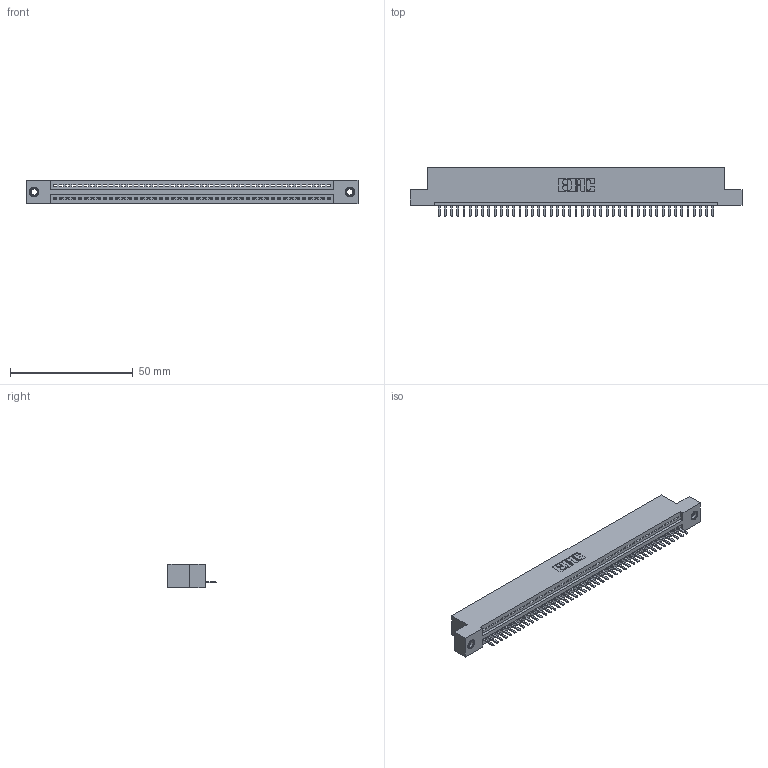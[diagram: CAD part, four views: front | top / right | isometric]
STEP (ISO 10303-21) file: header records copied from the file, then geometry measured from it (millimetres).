
FILE_DESCRIPTION (( 'STEP AP203' ), '1' );
FILE_NAME ('395-045-520-107.STEP', '2019-10-22T17:28:25', ( '' ), ( '' ), 'SwSTEP 2.0', 'SolidWorks 2016', '' );
FILE_SCHEMA (( 'CONFIG_CONTROL_DESIGN' ));
Length unit declared in the file: inch
Products named in the file (4): 345-292-001_345-293-120; 345 Part_Flush Mounting Lugs - 0.156 Dia-TI; 345-250-001_345-250-005-103; 395-045-520-107
Assembly tree (48 placements, depth 2):
  395-045-520-107
    345 Part_Flush Mounting Lugs - 0.156 Dia-TI
    345-292-001_345-293-120  x45
    345-250-001_345-250-005-103  x2
Bounding box: 135.51 x 19.68 x 9.4 mm (x, y, z)
Volume: 12752.4 mm3; surface area: 16596.6 mm2
Topology: 48 solids, 48 shells, 2976 faces, 8757 edges, 5710 vertices
Faces by surface type: plane 2002, cylinder 958, cone 12, torus 4
Entity records: 34764 total; most frequent: CARTESIAN_POINT 6014, ORIENTED_EDGE 5974, DIRECTION 5263, EDGE_CURVE 2987, VECTOR 2651, LINE 2651, VERTEX_POINT 1984, AXIS2_PLACEMENT_3D 1306
